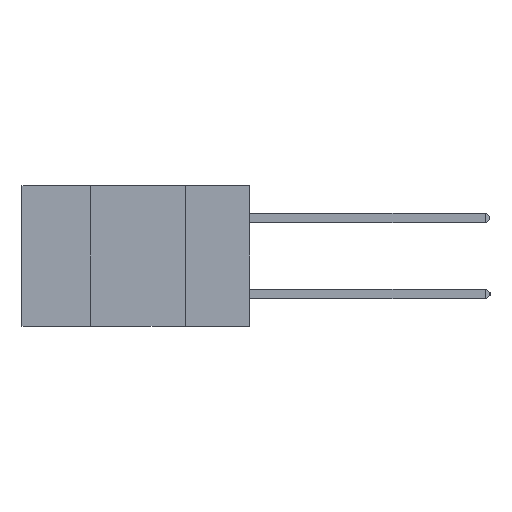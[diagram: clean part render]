
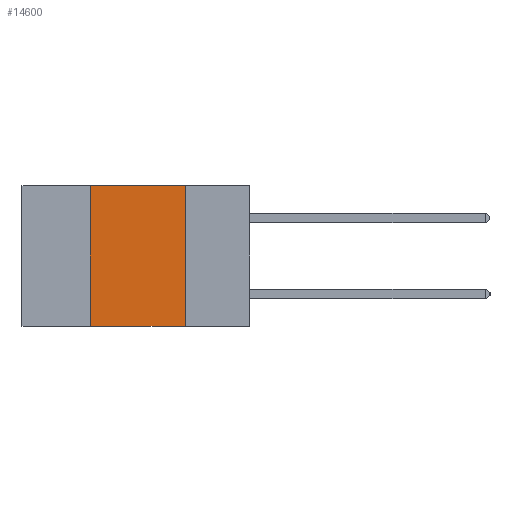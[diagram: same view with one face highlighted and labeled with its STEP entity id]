
A CAD part, left-side view. The second image highlights one B-rep face of the part: STEP entity #14600.
In plain terms, the highlighted planar face has unit normal (-1, 0, 0).
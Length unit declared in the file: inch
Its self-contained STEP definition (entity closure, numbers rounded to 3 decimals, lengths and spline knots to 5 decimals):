
#107 = CARTESIAN_POINT ( 'NONE',  ( 0., 0.6, 0. ) ) ;
#504 = VECTOR ( 'NONE', #4686, 39.37008 ) ;
#694 = DIRECTION ( 'NONE',  ( 0., -1., 0. ) ) ;
#1194 = DIRECTION ( 'NONE',  ( 0., -1., 0. ) ) ;
#1337 = ORIENTED_EDGE ( 'NONE', *, *, #6442, .T. ) ;
#1349 = DIRECTION ( 'NONE',  ( 1., 0., 0. ) ) ;
#2242 = CARTESIAN_POINT ( 'NONE',  ( 0., 0.17, 0. ) ) ;
#3286 = CARTESIAN_POINT ( 'NONE',  ( 0., 0.17, -0.37 ) ) ;
#3568 = VERTEX_POINT ( 'NONE', #12543 ) ;
#3748 = VECTOR ( 'NONE', #9134, 39.37008 ) ;
#4557 = EDGE_CURVE ( 'NONE', #6428, #12357, #6203, .T. ) ;
#4686 = DIRECTION ( 'NONE',  ( 0., 0., -1. ) ) ;
#4888 = ORIENTED_EDGE ( 'NONE', *, *, #4557, .F. ) ;
#4961 = VECTOR ( 'NONE', #694, 39.37008 ) ;
#6067 = ORIENTED_EDGE ( 'NONE', *, *, #9797, .F. ) ;
#6203 = LINE ( 'NONE', #13230, #4961 ) ;
#6428 = VERTEX_POINT ( 'NONE', #12582 ) ;
#6442 = EDGE_CURVE ( 'NONE', #3568, #8935, #13261, .T. ) ;
#8935 = VERTEX_POINT ( 'NONE', #3286 ) ;
#9134 = DIRECTION ( 'NONE',  ( 0., 0., 1. ) ) ;
#9713 = EDGE_CURVE ( 'NONE', #12357, #8935, #10137, .T. ) ;
#9717 = FACE_OUTER_BOUND ( 'NONE', #13350, .T. ) ;
#9785 = LINE ( 'NONE', #12431, #3748 ) ;
#9797 = EDGE_CURVE ( 'NONE', #3568, #6428, #9785, .T. ) ;
#10137 = LINE ( 'NONE', #2242, #504 ) ;
#11102 = ORIENTED_EDGE ( 'NONE', *, *, #9713, .F. ) ;
#11364 = CARTESIAN_POINT ( 'NONE',  ( 0., 0.6, -0.37 ) ) ;
#12357 = VERTEX_POINT ( 'NONE', #13082 ) ;
#12431 = CARTESIAN_POINT ( 'NONE',  ( 0., 0.42, 0. ) ) ;
#12543 = CARTESIAN_POINT ( 'NONE',  ( 0., 0.42, -0.37 ) ) ;
#12582 = CARTESIAN_POINT ( 'NONE',  ( 0., 0.42, 0. ) ) ;
#13082 = CARTESIAN_POINT ( 'NONE',  ( 0., 0.17, 0. ) ) ;
#13230 = CARTESIAN_POINT ( 'NONE',  ( 0., 0.6, 0. ) ) ;
#13261 = LINE ( 'NONE', #11364, #14710 ) ;
#13350 = EDGE_LOOP ( 'NONE', ( #11102, #4888, #6067, #1337 ) ) ;
#13448 = AXIS2_PLACEMENT_3D ( 'NONE', #107, #1349, #13806 ) ;
#13653 = PLANE ( 'NONE',  #13448 ) ;
#13806 = DIRECTION ( 'NONE',  ( 0., 0., -1. ) ) ;
#14600 = ADVANCED_FACE ( 'NONE', ( #9717 ), #13653, .F. ) ;
#14710 = VECTOR ( 'NONE', #1194, 39.37008 ) ;
